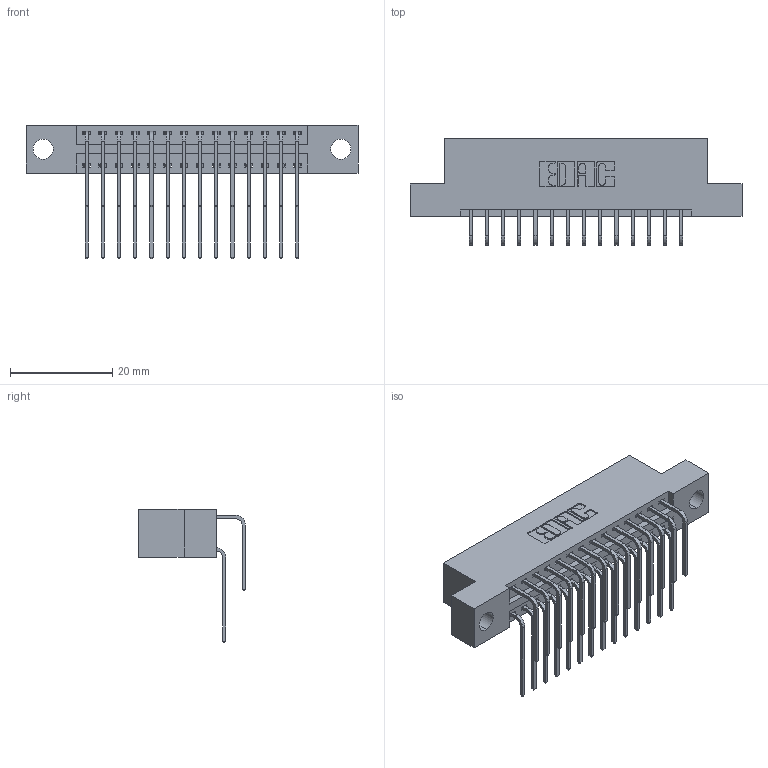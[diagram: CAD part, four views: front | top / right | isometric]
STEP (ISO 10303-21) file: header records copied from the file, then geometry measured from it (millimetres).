
FILE_DESCRIPTION (( 'STEP AP203' ), '1' );
FILE_NAME ('396-028-559-204.STEP', '2018-09-05T04:26:51', ( '' ), ( '' ), 'SwSTEP 2.0', 'SolidWorks 2016', '' );
FILE_SCHEMA (( 'CONFIG_CONTROL_DESIGN' ));
Length unit declared in the file: inch
Products named in the file (4): 346 Part_Flush Mounting Lugs - 0.156 Dia-TH; 345-292-001_558 559 Tail - 1; 345-292-001_559 Tail - 2; 396-028-559-204
Assembly tree (29 placements, depth 2):
  396-028-559-204
    346 Part_Flush Mounting Lugs - 0.156 Dia-TH
    345-292-001_558 559 Tail - 1  x14
    345-292-001_559 Tail - 2  x14
Bounding box: 65.02 x 20.89 x 26.16 mm (x, y, z)
Volume: 6196.8 mm3; surface area: 8666.1 mm2
Topology: 29 solids, 29 shells, 1634 faces, 4837 edges, 3186 vertices
Faces by surface type: plane 1112, cylinder 522
Entity records: 14693 total; most frequent: CARTESIAN_POINT 2511, ORIENTED_EDGE 2394, DIRECTION 2237, EDGE_CURVE 1197, VECTOR 969, LINE 969, VERTEX_POINT 794, AXIS2_PLACEMENT_3D 634
